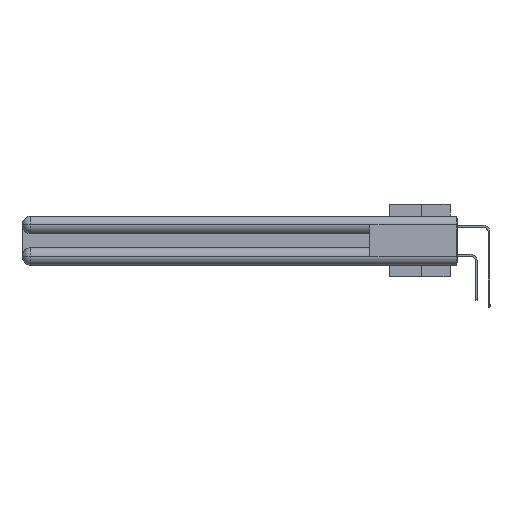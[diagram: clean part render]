
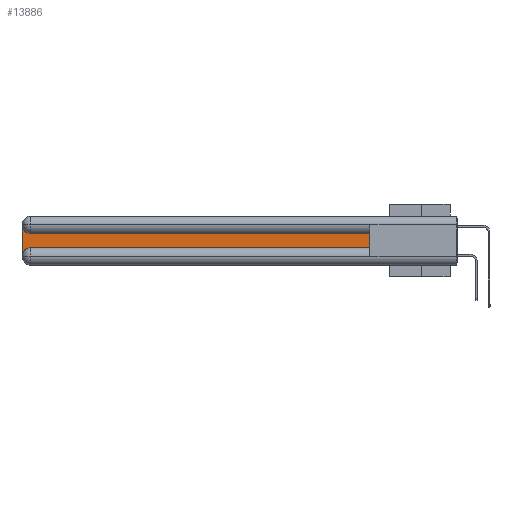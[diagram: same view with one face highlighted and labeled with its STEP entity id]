
A CAD part, left-side view. The second image highlights one B-rep face of the part: STEP entity #13886.
In plain terms, the highlighted planar face has unit normal (-1, 0, 0).
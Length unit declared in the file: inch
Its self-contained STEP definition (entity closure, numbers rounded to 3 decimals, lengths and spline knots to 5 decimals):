
#214 = DIRECTION ( 'NONE',  ( 0., 0., -1. ) ) ;
#1015 = ORIENTED_EDGE ( 'NONE', *, *, #15289, .T. ) ;
#2777 = LINE ( 'NONE', #28970, #25996 ) ;
#2985 = VECTOR ( 'NONE', #18234, 39.37008 ) ;
#3074 = CIRCLE ( 'NONE', #38594, 0.06 ) ;
#5046 = CARTESIAN_POINT ( 'NONE',  ( 0.075, 3., -0.2775 ) ) ;
#5225 = DIRECTION ( 'NONE',  ( 1., 0., 0. ) ) ;
#7949 = ORIENTED_EDGE ( 'NONE', *, *, #39221, .T. ) ;
#8056 = VERTEX_POINT ( 'NONE', #5046 ) ;
#9109 = VERTEX_POINT ( 'NONE', #38075 ) ;
#10378 = CIRCLE ( 'NONE', #11766, 0.06 ) ;
#10654 = EDGE_CURVE ( 'NONE', #38995, #20389, #23920, .T. ) ;
#11109 = CARTESIAN_POINT ( 'NONE',  ( 0.075, 0.6, -0.2175 ) ) ;
#11628 = EDGE_CURVE ( 'NONE', #8056, #9109, #10378, .T. ) ;
#11766 = AXIS2_PLACEMENT_3D ( 'NONE', #24570, #39867, #33384 ) ;
#13400 = VERTEX_POINT ( 'NONE', #14203 ) ;
#13865 = DIRECTION ( 'NONE',  ( 0., 1., 0. ) ) ;
#13886 = ADVANCED_FACE ( 'NONE', ( #32705 ), #33982, .F. ) ;
#14174 = DIRECTION ( 'NONE',  ( 0., -1., 0. ) ) ;
#14203 = CARTESIAN_POINT ( 'NONE',  ( 0.075, 2.94, -0.1225 ) ) ;
#14683 = VECTOR ( 'NONE', #14174, 39.37008 ) ;
#15289 = EDGE_CURVE ( 'NONE', #20389, #13400, #29816, .T. ) ;
#15622 = CARTESIAN_POINT ( 'NONE',  ( 0.075, 2.94, -0.0625 ) ) ;
#18026 = CARTESIAN_POINT ( 'NONE',  ( 0.075, 0.6, -0.1225 ) ) ;
#18234 = DIRECTION ( 'NONE',  ( 0., 0., 1. ) ) ;
#19190 = ORIENTED_EDGE ( 'NONE', *, *, #32739, .T. ) ;
#19711 = AXIS2_PLACEMENT_3D ( 'NONE', #26813, #5225, #39424 ) ;
#19965 = CARTESIAN_POINT ( 'NONE',  ( 0.075, 0.6, -0.1225 ) ) ;
#20389 = VERTEX_POINT ( 'NONE', #18026 ) ;
#21135 = ORIENTED_EDGE ( 'NONE', *, *, #36760, .T. ) ;
#23920 = LINE ( 'NONE', #11109, #2985 ) ;
#24570 = CARTESIAN_POINT ( 'NONE',  ( 0.075, 2.94, -0.2775 ) ) ;
#25726 = VERTEX_POINT ( 'NONE', #28771 ) ;
#25996 = VECTOR ( 'NONE', #214, 39.37008 ) ;
#26813 = CARTESIAN_POINT ( 'NONE',  ( 0.075, 3., -0.1225 ) ) ;
#27416 = LINE ( 'NONE', #30765, #14683 ) ;
#27870 = ORIENTED_EDGE ( 'NONE', *, *, #10654, .T. ) ;
#28421 = DIRECTION ( 'NONE',  ( 0., 0., -1. ) ) ;
#28627 = DIRECTION ( 'NONE',  ( 1., 0., 0. ) ) ;
#28771 = CARTESIAN_POINT ( 'NONE',  ( 0.075, 3., -0.0625 ) ) ;
#28970 = CARTESIAN_POINT ( 'NONE',  ( 0.075, 3., -0.2175 ) ) ;
#29470 = ORIENTED_EDGE ( 'NONE', *, *, #11628, .T. ) ;
#29816 = LINE ( 'NONE', #19965, #34616 ) ;
#30765 = CARTESIAN_POINT ( 'NONE',  ( 0.075, 0.6, -0.2175 ) ) ;
#32705 = FACE_OUTER_BOUND ( 'NONE', #38057, .T. ) ;
#32739 = EDGE_CURVE ( 'NONE', #13400, #25726, #3074, .T. ) ;
#33384 = DIRECTION ( 'NONE',  ( 0., 0., -1. ) ) ;
#33982 = PLANE ( 'NONE',  #19711 ) ;
#34616 = VECTOR ( 'NONE', #13865, 39.37008 ) ;
#36760 = EDGE_CURVE ( 'NONE', #25726, #8056, #2777, .T. ) ;
#38057 = EDGE_LOOP ( 'NONE', ( #1015, #19190, #21135, #29470, #7949, #27870 ) ) ;
#38075 = CARTESIAN_POINT ( 'NONE',  ( 0.075, 2.94, -0.2175 ) ) ;
#38549 = CARTESIAN_POINT ( 'NONE',  ( 0.075, 0.6, -0.2175 ) ) ;
#38594 = AXIS2_PLACEMENT_3D ( 'NONE', #15622, #28627, #28421 ) ;
#38995 = VERTEX_POINT ( 'NONE', #38549 ) ;
#39221 = EDGE_CURVE ( 'NONE', #9109, #38995, #27416, .T. ) ;
#39424 = DIRECTION ( 'NONE',  ( 0., 0., -1. ) ) ;
#39867 = DIRECTION ( 'NONE',  ( 1., 0., 0. ) ) ;
